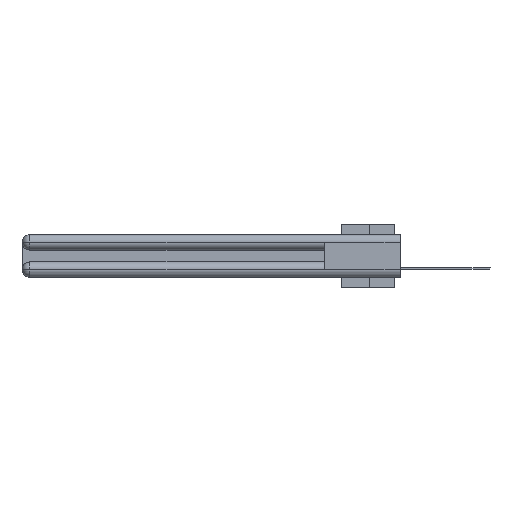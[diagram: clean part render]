
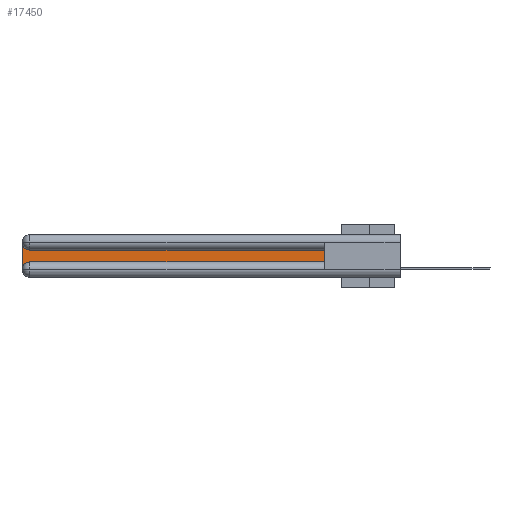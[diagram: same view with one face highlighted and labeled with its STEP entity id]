
A CAD part, left-side view. The second image highlights one B-rep face of the part: STEP entity #17450.
In plain terms, the highlighted planar face has unit normal (-1, 0, 0).
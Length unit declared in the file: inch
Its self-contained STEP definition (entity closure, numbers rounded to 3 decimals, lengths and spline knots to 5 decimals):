
#657 = CARTESIAN_POINT ( 'NONE',  ( 0.075, 3., -0.0625 ) ) ;
#1494 = ORIENTED_EDGE ( 'NONE', *, *, #9304, .T. ) ;
#1680 = DIRECTION ( 'NONE',  ( 1., 0., 0. ) ) ;
#1886 = LINE ( 'NONE', #6143, #2821 ) ;
#2821 = VECTOR ( 'NONE', #6267, 39.37008 ) ;
#3475 = ORIENTED_EDGE ( 'NONE', *, *, #22183, .T. ) ;
#3906 = VERTEX_POINT ( 'NONE', #36268 ) ;
#5271 = CIRCLE ( 'NONE', #34267, 0.06 ) ;
#5568 = CARTESIAN_POINT ( 'NONE',  ( 0.075, 3., -0.2175 ) ) ;
#6143 = CARTESIAN_POINT ( 'NONE',  ( 0.075, 0.6, -0.2175 ) ) ;
#6267 = DIRECTION ( 'NONE',  ( 0., -1., 0. ) ) ;
#8116 = LINE ( 'NONE', #34199, #24904 ) ;
#8490 = CIRCLE ( 'NONE', #26632, 0.06 ) ;
#9304 = EDGE_CURVE ( 'NONE', #10224, #17364, #8116, .T. ) ;
#10224 = VERTEX_POINT ( 'NONE', #37683 ) ;
#10853 = ORIENTED_EDGE ( 'NONE', *, *, #33320, .T. ) ;
#10903 = DIRECTION ( 'NONE',  ( 0., 1., 0. ) ) ;
#11470 = EDGE_CURVE ( 'NONE', #37835, #3906, #20569, .T. ) ;
#12088 = DIRECTION ( 'NONE',  ( 0., 0., -1. ) ) ;
#12335 = DIRECTION ( 'NONE',  ( 1., 0., 0. ) ) ;
#12642 = VECTOR ( 'NONE', #26242, 39.37008 ) ;
#14816 = CARTESIAN_POINT ( 'NONE',  ( 0.075, 2.94, -0.1225 ) ) ;
#17364 = VERTEX_POINT ( 'NONE', #29980 ) ;
#17450 = ADVANCED_FACE ( 'NONE', ( #36707 ), #27633, .F. ) ;
#18663 = DIRECTION ( 'NONE',  ( 0., 0., -1. ) ) ;
#20569 = LINE ( 'NONE', #5568, #12642 ) ;
#20850 = VECTOR ( 'NONE', #10903, 39.37008 ) ;
#21291 = AXIS2_PLACEMENT_3D ( 'NONE', #36365, #33480, #18663 ) ;
#22183 = EDGE_CURVE ( 'NONE', #38191, #10224, #1886, .T. ) ;
#22913 = EDGE_CURVE ( 'NONE', #17364, #29943, #25517, .T. ) ;
#24904 = VECTOR ( 'NONE', #37222, 39.37008 ) ;
#25517 = LINE ( 'NONE', #34568, #20850 ) ;
#26242 = DIRECTION ( 'NONE',  ( 0., 0., -1. ) ) ;
#26632 = AXIS2_PLACEMENT_3D ( 'NONE', #31605, #1680, #31338 ) ;
#27044 = CARTESIAN_POINT ( 'NONE',  ( 0.075, 2.94, -0.2775 ) ) ;
#27633 = PLANE ( 'NONE',  #21291 ) ;
#28100 = EDGE_CURVE ( 'NONE', #3906, #38191, #5271, .T. ) ;
#29454 = ORIENTED_EDGE ( 'NONE', *, *, #11470, .T. ) ;
#29943 = VERTEX_POINT ( 'NONE', #14816 ) ;
#29980 = CARTESIAN_POINT ( 'NONE',  ( 0.075, 0.6, -0.1225 ) ) ;
#31171 = EDGE_LOOP ( 'NONE', ( #37287, #10853, #29454, #32220, #3475, #1494 ) ) ;
#31338 = DIRECTION ( 'NONE',  ( 0., 0., -1. ) ) ;
#31605 = CARTESIAN_POINT ( 'NONE',  ( 0.075, 2.94, -0.0625 ) ) ;
#32220 = ORIENTED_EDGE ( 'NONE', *, *, #28100, .T. ) ;
#33320 = EDGE_CURVE ( 'NONE', #29943, #37835, #8490, .T. ) ;
#33480 = DIRECTION ( 'NONE',  ( 1., 0., 0. ) ) ;
#34199 = CARTESIAN_POINT ( 'NONE',  ( 0.075, 0.6, -0.2175 ) ) ;
#34267 = AXIS2_PLACEMENT_3D ( 'NONE', #27044, #12335, #12088 ) ;
#34568 = CARTESIAN_POINT ( 'NONE',  ( 0.075, 0.6, -0.1225 ) ) ;
#34986 = CARTESIAN_POINT ( 'NONE',  ( 0.075, 2.94, -0.2175 ) ) ;
#36268 = CARTESIAN_POINT ( 'NONE',  ( 0.075, 3., -0.2775 ) ) ;
#36365 = CARTESIAN_POINT ( 'NONE',  ( 0.075, 3., -0.1225 ) ) ;
#36707 = FACE_OUTER_BOUND ( 'NONE', #31171, .T. ) ;
#37222 = DIRECTION ( 'NONE',  ( 0., 0., 1. ) ) ;
#37287 = ORIENTED_EDGE ( 'NONE', *, *, #22913, .T. ) ;
#37683 = CARTESIAN_POINT ( 'NONE',  ( 0.075, 0.6, -0.2175 ) ) ;
#37835 = VERTEX_POINT ( 'NONE', #657 ) ;
#38191 = VERTEX_POINT ( 'NONE', #34986 ) ;
